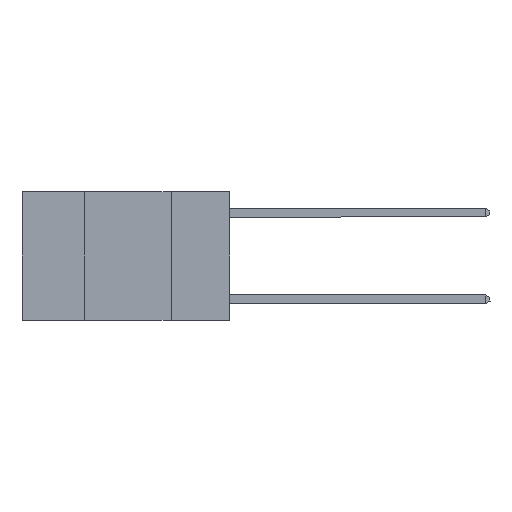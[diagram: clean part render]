
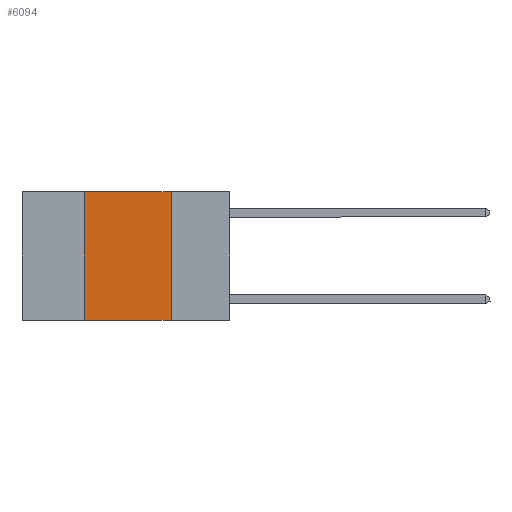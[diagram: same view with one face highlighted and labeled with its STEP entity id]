
A CAD part, left-side view. The second image highlights one B-rep face of the part: STEP entity #6094.
In plain terms, the highlighted planar face has unit normal (-1, 0, 0).
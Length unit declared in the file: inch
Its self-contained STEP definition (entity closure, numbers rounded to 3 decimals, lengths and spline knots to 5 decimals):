
#211 = LINE ( 'NONE', #9151, #2240 ) ;
#874 = EDGE_CURVE ( 'NONE', #4275, #8820, #8463, .T. ) ;
#1224 = DIRECTION ( 'NONE',  ( 0., 0., 1. ) ) ;
#1361 = CARTESIAN_POINT ( 'NONE',  ( 0., 0.6, 0. ) ) ;
#1690 = ORIENTED_EDGE ( 'NONE', *, *, #874, .T. ) ;
#1768 = CARTESIAN_POINT ( 'NONE',  ( 0., 0.42, -0.37 ) ) ;
#1799 = ORIENTED_EDGE ( 'NONE', *, *, #3865, .F. ) ;
#2239 = DIRECTION ( 'NONE',  ( 0., 0., -1. ) ) ;
#2240 = VECTOR ( 'NONE', #9973, 39.37008 ) ;
#2936 = CARTESIAN_POINT ( 'NONE',  ( 0., 0.42, 0. ) ) ;
#3116 = DIRECTION ( 'NONE',  ( 0., 0., -1. ) ) ;
#3153 = VECTOR ( 'NONE', #2239, 39.37008 ) ;
#3695 = EDGE_CURVE ( 'NONE', #10108, #10174, #211, .T. ) ;
#3816 = ORIENTED_EDGE ( 'NONE', *, *, #3695, .F. ) ;
#3846 = CARTESIAN_POINT ( 'NONE',  ( 0., 0.17, 0. ) ) ;
#3858 = EDGE_LOOP ( 'NONE', ( #1799, #3816, #5833, #1690 ) ) ;
#3865 = EDGE_CURVE ( 'NONE', #10174, #8820, #10162, .T. ) ;
#4061 = FACE_OUTER_BOUND ( 'NONE', #3858, .T. ) ;
#4275 = VERTEX_POINT ( 'NONE', #1768 ) ;
#4637 = CARTESIAN_POINT ( 'NONE',  ( 0., 0.42, 0. ) ) ;
#5679 = PLANE ( 'NONE',  #8872 ) ;
#5833 = ORIENTED_EDGE ( 'NONE', *, *, #10146, .F. ) ;
#5964 = VECTOR ( 'NONE', #11112, 39.37008 ) ;
#6094 = ADVANCED_FACE ( 'NONE', ( #4061 ), #5679, .F. ) ;
#6703 = CARTESIAN_POINT ( 'NONE',  ( 0., 0.17, -0.37 ) ) ;
#7937 = LINE ( 'NONE', #2936, #9943 ) ;
#8463 = LINE ( 'NONE', #10561, #5964 ) ;
#8485 = DIRECTION ( 'NONE',  ( 1., 0., 0. ) ) ;
#8820 = VERTEX_POINT ( 'NONE', #6703 ) ;
#8872 = AXIS2_PLACEMENT_3D ( 'NONE', #1361, #8485, #3116 ) ;
#9151 = CARTESIAN_POINT ( 'NONE',  ( 0., 0.6, 0. ) ) ;
#9943 = VECTOR ( 'NONE', #1224, 39.37008 ) ;
#9973 = DIRECTION ( 'NONE',  ( 0., -1., 0. ) ) ;
#10107 = CARTESIAN_POINT ( 'NONE',  ( 0., 0.17, 0. ) ) ;
#10108 = VERTEX_POINT ( 'NONE', #4637 ) ;
#10146 = EDGE_CURVE ( 'NONE', #4275, #10108, #7937, .T. ) ;
#10162 = LINE ( 'NONE', #10107, #3153 ) ;
#10174 = VERTEX_POINT ( 'NONE', #3846 ) ;
#10561 = CARTESIAN_POINT ( 'NONE',  ( 0., 0.6, -0.37 ) ) ;
#11112 = DIRECTION ( 'NONE',  ( 0., -1., 0. ) ) ;
